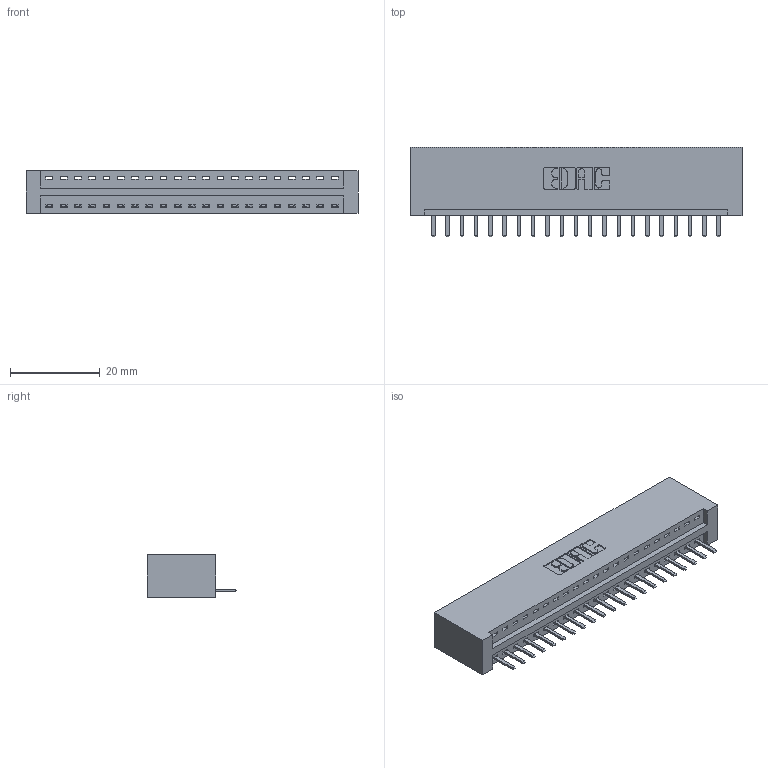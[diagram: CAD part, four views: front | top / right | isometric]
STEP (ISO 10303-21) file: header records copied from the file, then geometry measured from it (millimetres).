
FILE_DESCRIPTION (( 'STEP AP203' ), '1' );
FILE_NAME ('346-021-520-101.STEP', '2018-08-20T22:39:24', ( '' ), ( '' ), 'SwSTEP 2.0', 'SolidWorks 2016', '' );
FILE_SCHEMA (( 'CONFIG_CONTROL_DESIGN' ));
Length unit declared in the file: inch
Products named in the file (3): 346 Part_No Mounting Lugs; 345-292-001_345-293-120; 346-021-520-101
Assembly tree (22 placements, depth 2):
  346-021-520-101
    346 Part_No Mounting Lugs
    345-292-001_345-293-120  x21
Bounding box: 73.91 x 20.02 x 9.4 mm (x, y, z)
Volume: 7419.5 mm3; surface area: 8920.3 mm2
Topology: 22 solids, 22 shells, 1416 faces, 4169 edges, 2722 vertices
Faces by surface type: plane 954, cylinder 462
Entity records: 15697 total; most frequent: CARTESIAN_POINT 2715, ORIENTED_EDGE 2658, DIRECTION 2403, EDGE_CURVE 1329, LINE 1117, VECTOR 1117, VERTEX_POINT 882, AXIS2_PLACEMENT_3D 643
